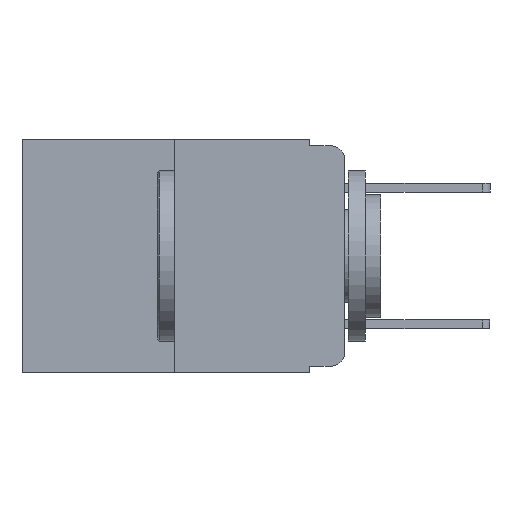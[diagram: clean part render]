
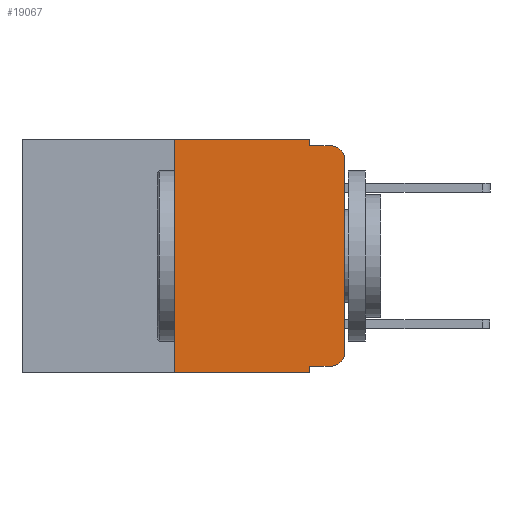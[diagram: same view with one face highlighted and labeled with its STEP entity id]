
A CAD part, left-side view. The second image highlights one B-rep face of the part: STEP entity #19067.
In plain terms, the highlighted planar face has unit normal (-1, 0, 0).
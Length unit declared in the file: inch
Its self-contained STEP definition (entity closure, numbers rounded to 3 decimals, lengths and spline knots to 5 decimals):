
#117 = CARTESIAN_POINT ( 'NONE',  ( 0., 0.051, 0. ) ) ;
#271 = EDGE_CURVE ( 'NONE', #7669, #10776, #13175, .T. ) ;
#617 = VERTEX_POINT ( 'NONE', #6267 ) ;
#930 = VECTOR ( 'NONE', #7293, 39.37008 ) ;
#1066 = EDGE_CURVE ( 'NONE', #13671, #5848, #2466, .T. ) ;
#1166 = EDGE_CURVE ( 'NONE', #10776, #13597, #11837, .T. ) ;
#1500 = CARTESIAN_POINT ( 'NONE',  ( 0., 0.02, -0.313 ) ) ;
#1516 = DIRECTION ( 'NONE',  ( 0., 0., -1. ) ) ;
#1533 = EDGE_CURVE ( 'NONE', #13671, #7669, #13602, .T. ) ;
#2242 = CARTESIAN_POINT ( 'NONE',  ( 0., 0.25, -0.343 ) ) ;
#2466 = LINE ( 'NONE', #8598, #17034 ) ;
#2538 = LINE ( 'NONE', #10524, #17093 ) ;
#2615 = EDGE_CURVE ( 'NONE', #9722, #4098, #15635, .T. ) ;
#2616 = VERTEX_POINT ( 'NONE', #14339 ) ;
#2673 = VECTOR ( 'NONE', #19486, 39.37008 ) ;
#2798 = ORIENTED_EDGE ( 'NONE', *, *, #15182, .F. ) ;
#2895 = CARTESIAN_POINT ( 'NONE',  ( 0., 0.02, -0.333 ) ) ;
#3627 = ORIENTED_EDGE ( 'NONE', *, *, #1066, .T. ) ;
#4098 = VERTEX_POINT ( 'NONE', #9114 ) ;
#4122 = ORIENTED_EDGE ( 'NONE', *, *, #1166, .F. ) ;
#4250 = AXIS2_PLACEMENT_3D ( 'NONE', #9244, #19318, #10692 ) ;
#4503 = EDGE_CURVE ( 'NONE', #2616, #9722, #16015, .T. ) ;
#4672 = ORIENTED_EDGE ( 'NONE', *, *, #4503, .T. ) ;
#4691 = FACE_OUTER_BOUND ( 'NONE', #5864, .T. ) ;
#5223 = AXIS2_PLACEMENT_3D ( 'NONE', #1500, #18086, #8503 ) ;
#5848 = VERTEX_POINT ( 'NONE', #7923 ) ;
#5864 = EDGE_LOOP ( 'NONE', ( #16179, #10102, #2798, #4122, #8743, #10791, #3627, #14643, #4672, #17372 ) ) ;
#6267 = CARTESIAN_POINT ( 'NONE',  ( 0., 0.02, -0.01 ) ) ;
#6531 = DIRECTION ( 'NONE',  ( 0., 0., -1. ) ) ;
#7132 = LINE ( 'NONE', #8063, #14416 ) ;
#7293 = DIRECTION ( 'NONE',  ( 0., -1., 0. ) ) ;
#7552 = DIRECTION ( 'NONE',  ( 0., -1., 0. ) ) ;
#7669 = VERTEX_POINT ( 'NONE', #13369 ) ;
#7904 = CARTESIAN_POINT ( 'NONE',  ( 0., 0.02, -0.03 ) ) ;
#7923 = CARTESIAN_POINT ( 'NONE',  ( 0., 0.051, -0.343 ) ) ;
#8063 = CARTESIAN_POINT ( 'NONE',  ( 0., 0.051, 0. ) ) ;
#8503 = DIRECTION ( 'NONE',  ( 0., 0., -1. ) ) ;
#8598 = CARTESIAN_POINT ( 'NONE',  ( 0., 0.473, -0.343 ) ) ;
#8743 = ORIENTED_EDGE ( 'NONE', *, *, #271, .F. ) ;
#8746 = CARTESIAN_POINT ( 'NONE',  ( 0., 0., -0.03 ) ) ;
#9114 = CARTESIAN_POINT ( 'NONE',  ( 0., 0., -0.313 ) ) ;
#9130 = EDGE_CURVE ( 'NONE', #4098, #11896, #10874, .T. ) ;
#9244 = CARTESIAN_POINT ( 'NONE',  ( 0., 0.473, 0. ) ) ;
#9329 = VECTOR ( 'NONE', #18887, 39.37008 ) ;
#9402 = CARTESIAN_POINT ( 'NONE',  ( 0., 0., 0. ) ) ;
#9405 = DIRECTION ( 'NONE',  ( 0., 0., -1. ) ) ;
#9722 = VERTEX_POINT ( 'NONE', #2895 ) ;
#10102 = ORIENTED_EDGE ( 'NONE', *, *, #10916, .T. ) ;
#10495 = CARTESIAN_POINT ( 'NONE',  ( 0., 0.051, 0. ) ) ;
#10524 = CARTESIAN_POINT ( 'NONE',  ( 0., 0.051, -0.01 ) ) ;
#10692 = DIRECTION ( 'NONE',  ( 0., 0., -1. ) ) ;
#10776 = VERTEX_POINT ( 'NONE', #10495 ) ;
#10791 = ORIENTED_EDGE ( 'NONE', *, *, #1533, .F. ) ;
#10874 = LINE ( 'NONE', #9402, #2673 ) ;
#10916 = EDGE_CURVE ( 'NONE', #11896, #617, #14631, .T. ) ;
#11729 = CARTESIAN_POINT ( 'NONE',  ( 0., 0.473, 0. ) ) ;
#11837 = LINE ( 'NONE', #117, #18602 ) ;
#11896 = VERTEX_POINT ( 'NONE', #8746 ) ;
#12264 = DIRECTION ( 'NONE',  ( 0., -1., 0. ) ) ;
#12589 = VECTOR ( 'NONE', #16572, 39.37008 ) ;
#13175 = LINE ( 'NONE', #11729, #930 ) ;
#13369 = CARTESIAN_POINT ( 'NONE',  ( 0., 0.25, 0. ) ) ;
#13597 = VERTEX_POINT ( 'NONE', #14174 ) ;
#13602 = LINE ( 'NONE', #16216, #9329 ) ;
#13671 = VERTEX_POINT ( 'NONE', #2242 ) ;
#14081 = EDGE_CURVE ( 'NONE', #2616, #5848, #7132, .T. ) ;
#14094 = AXIS2_PLACEMENT_3D ( 'NONE', #7904, #18054, #9405 ) ;
#14174 = CARTESIAN_POINT ( 'NONE',  ( 0., 0.051, -0.01 ) ) ;
#14339 = CARTESIAN_POINT ( 'NONE',  ( 0., 0.051, -0.333 ) ) ;
#14416 = VECTOR ( 'NONE', #6531, 39.37008 ) ;
#14631 = CIRCLE ( 'NONE', #14094, 0.02 ) ;
#14643 = ORIENTED_EDGE ( 'NONE', *, *, #14081, .F. ) ;
#15182 = EDGE_CURVE ( 'NONE', #13597, #617, #2538, .T. ) ;
#15635 = CIRCLE ( 'NONE', #5223, 0.02 ) ;
#16015 = LINE ( 'NONE', #16465, #12589 ) ;
#16179 = ORIENTED_EDGE ( 'NONE', *, *, #9130, .T. ) ;
#16216 = CARTESIAN_POINT ( 'NONE',  ( 0., 0.25, 0. ) ) ;
#16432 = PLANE ( 'NONE',  #4250 ) ;
#16465 = CARTESIAN_POINT ( 'NONE',  ( 0., 0.051, -0.333 ) ) ;
#16572 = DIRECTION ( 'NONE',  ( 0., -1., 0. ) ) ;
#17034 = VECTOR ( 'NONE', #12264, 39.37008 ) ;
#17093 = VECTOR ( 'NONE', #7552, 39.37008 ) ;
#17372 = ORIENTED_EDGE ( 'NONE', *, *, #2615, .T. ) ;
#18054 = DIRECTION ( 'NONE',  ( -1., 0., 0. ) ) ;
#18086 = DIRECTION ( 'NONE',  ( -1., 0., 0. ) ) ;
#18602 = VECTOR ( 'NONE', #1516, 39.37008 ) ;
#18887 = DIRECTION ( 'NONE',  ( 0., 0., 1. ) ) ;
#19067 = ADVANCED_FACE ( 'NONE', ( #4691 ), #16432, .F. ) ;
#19318 = DIRECTION ( 'NONE',  ( 1., 0., 0. ) ) ;
#19486 = DIRECTION ( 'NONE',  ( 0., 0., 1. ) ) ;
